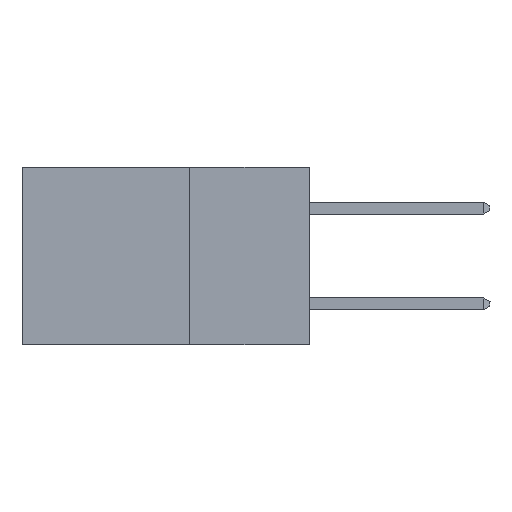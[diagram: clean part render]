
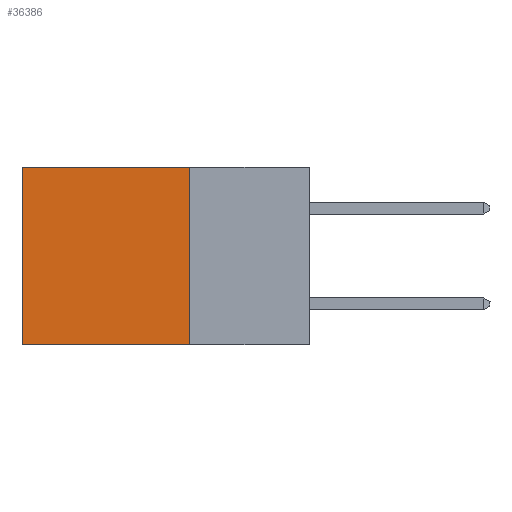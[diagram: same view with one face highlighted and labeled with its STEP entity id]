
A CAD part, left-side view. The second image highlights one B-rep face of the part: STEP entity #36386.
In plain terms, the highlighted planar face has unit normal (-1, 0, 0).
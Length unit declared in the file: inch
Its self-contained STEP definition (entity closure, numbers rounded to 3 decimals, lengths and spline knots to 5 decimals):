
#186 = DIRECTION ( 'NONE',  ( 0., 0., -1. ) ) ;
#486 = VECTOR ( 'NONE', #6630, 39.37008 ) ;
#1885 = LINE ( 'NONE', #12277, #11396 ) ;
#2331 = CARTESIAN_POINT ( 'NONE',  ( 0.2875, 0.25, 0. ) ) ;
#2888 = ORIENTED_EDGE ( 'NONE', *, *, #41902, .F. ) ;
#3003 = EDGE_CURVE ( 'NONE', #22491, #33712, #1885, .T. ) ;
#4117 = VERTEX_POINT ( 'NONE', #23949 ) ;
#5872 = LINE ( 'NONE', #11724, #7040 ) ;
#6630 = DIRECTION ( 'NONE',  ( 0., 1., 0. ) ) ;
#7040 = VECTOR ( 'NONE', #15111, 39.37008 ) ;
#8163 = CARTESIAN_POINT ( 'NONE',  ( 0.2875, 0.25, 0. ) ) ;
#9605 = VERTEX_POINT ( 'NONE', #30384 ) ;
#11396 = VECTOR ( 'NONE', #22622, 39.37008 ) ;
#11724 = CARTESIAN_POINT ( 'NONE',  ( 0.2875, 0.6, 0. ) ) ;
#12277 = CARTESIAN_POINT ( 'NONE',  ( 0.2875, 0.25, -0.37 ) ) ;
#15111 = DIRECTION ( 'NONE',  ( 0., 0., -1. ) ) ;
#18675 = CARTESIAN_POINT ( 'NONE',  ( 0.2875, 0.25, -0.37 ) ) ;
#18830 = EDGE_CURVE ( 'NONE', #9605, #4117, #39936, .T. ) ;
#18897 = ORIENTED_EDGE ( 'NONE', *, *, #18830, .T. ) ;
#20638 = EDGE_CURVE ( 'NONE', #4117, #33712, #5872, .T. ) ;
#20847 = DIRECTION ( 'NONE',  ( 0., 0., -1. ) ) ;
#21577 = EDGE_LOOP ( 'NONE', ( #29713, #28426, #2888, #18897 ) ) ;
#22491 = VERTEX_POINT ( 'NONE', #18675 ) ;
#22622 = DIRECTION ( 'NONE',  ( 0., 1., 0. ) ) ;
#23949 = CARTESIAN_POINT ( 'NONE',  ( 0.2875, 0.6, 0. ) ) ;
#24209 = PLANE ( 'NONE',  #28785 ) ;
#24303 = LINE ( 'NONE', #8163, #29075 ) ;
#27582 = DIRECTION ( 'NONE',  ( 1., 0., 0. ) ) ;
#28426 = ORIENTED_EDGE ( 'NONE', *, *, #3003, .F. ) ;
#28785 = AXIS2_PLACEMENT_3D ( 'NONE', #40651, #27582, #20847 ) ;
#29075 = VECTOR ( 'NONE', #186, 39.37008 ) ;
#29713 = ORIENTED_EDGE ( 'NONE', *, *, #20638, .T. ) ;
#30384 = CARTESIAN_POINT ( 'NONE',  ( 0.2875, 0.25, 0. ) ) ;
#31783 = CARTESIAN_POINT ( 'NONE',  ( 0.2875, 0.6, -0.37 ) ) ;
#33712 = VERTEX_POINT ( 'NONE', #31783 ) ;
#34767 = FACE_OUTER_BOUND ( 'NONE', #21577, .T. ) ;
#36386 = ADVANCED_FACE ( 'NONE', ( #34767 ), #24209, .F. ) ;
#39936 = LINE ( 'NONE', #2331, #486 ) ;
#40651 = CARTESIAN_POINT ( 'NONE',  ( 0.2875, 0.25, 0. ) ) ;
#41902 = EDGE_CURVE ( 'NONE', #9605, #22491, #24303, .T. ) ;
